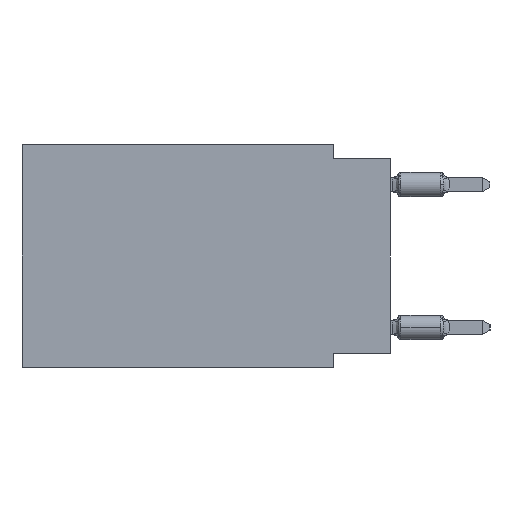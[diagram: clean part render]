
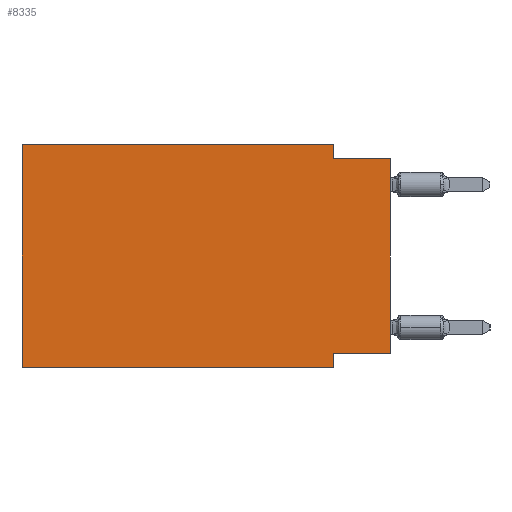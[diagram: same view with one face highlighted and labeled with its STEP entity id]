
A CAD part, left-side view. The second image highlights one B-rep face of the part: STEP entity #8335.
In plain terms, the highlighted planar face has unit normal (-1, 0, 0).
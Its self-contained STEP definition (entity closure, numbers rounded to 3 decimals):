
#845 = EDGE_CURVE ( 'NONE', #12443, #11943, #16083, .T. ) ;
#1323 = CARTESIAN_POINT ( 'NONE',  ( 0., 16.383, 0. ) ) ;
#2294 = EDGE_CURVE ( 'NONE', #23353, #10961, #6311, .T. ) ;
#3761 = VECTOR ( 'NONE', #19683, 1000. ) ;
#4020 = EDGE_CURVE ( 'NONE', #7304, #17691, #24039, .T. ) ;
#4338 = VECTOR ( 'NONE', #15937, 1000. ) ;
#4345 = EDGE_CURVE ( 'NONE', #23353, #12443, #23044, .T. ) ;
#4867 = CARTESIAN_POINT ( 'NONE',  ( 0., 2.54, -9.906 ) ) ;
#4906 = LINE ( 'NONE', #21512, #3761 ) ;
#5640 = EDGE_CURVE ( 'NONE', #17691, #22549, #6703, .T. ) ;
#6203 = ORIENTED_EDGE ( 'NONE', *, *, #845, .F. ) ;
#6311 = LINE ( 'NONE', #9970, #8726 ) ;
#6531 = EDGE_CURVE ( 'NONE', #10231, #10961, #4906, .T. ) ;
#6579 = ORIENTED_EDGE ( 'NONE', *, *, #4345, .F. ) ;
#6703 = LINE ( 'NONE', #17707, #21870 ) ;
#7304 = VERTEX_POINT ( 'NONE', #21574 ) ;
#8269 = ORIENTED_EDGE ( 'NONE', *, *, #5640, .F. ) ;
#8335 = ADVANCED_FACE ( 'NONE', ( #10735 ), #21973, .F. ) ;
#8495 = CARTESIAN_POINT ( 'NONE',  ( 0., 0., -9.271 ) ) ;
#8531 = AXIS2_PLACEMENT_3D ( 'NONE', #1323, #19904, #20152 ) ;
#8726 = VECTOR ( 'NONE', #17431, 1000. ) ;
#8880 = DIRECTION ( 'NONE',  ( 0., 0., 1. ) ) ;
#9063 = VECTOR ( 'NONE', #19872, 1000. ) ;
#9106 = EDGE_CURVE ( 'NONE', #7304, #11943, #16672, .T. ) ;
#9144 = EDGE_LOOP ( 'NONE', ( #17101, #19154, #11275, #8269, #10000, #17847, #6203, #6579 ) ) ;
#9970 = CARTESIAN_POINT ( 'NONE',  ( 0., 0., 0. ) ) ;
#10000 = ORIENTED_EDGE ( 'NONE', *, *, #4020, .F. ) ;
#10231 = VERTEX_POINT ( 'NONE', #10335 ) ;
#10335 = CARTESIAN_POINT ( 'NONE',  ( 0., 2.54, -0.635 ) ) ;
#10477 = DIRECTION ( 'NONE',  ( 0., -1., 0. ) ) ;
#10491 = CARTESIAN_POINT ( 'NONE',  ( 0., 16.383, 0. ) ) ;
#10735 = FACE_OUTER_BOUND ( 'NONE', #9144, .T. ) ;
#10957 = CARTESIAN_POINT ( 'NONE',  ( 0., 0., -9.271 ) ) ;
#10961 = VERTEX_POINT ( 'NONE', #11374 ) ;
#11225 = CARTESIAN_POINT ( 'NONE',  ( 0., 2.54, -9.271 ) ) ;
#11275 = ORIENTED_EDGE ( 'NONE', *, *, #22715, .F. ) ;
#11374 = CARTESIAN_POINT ( 'NONE',  ( 0., 0., -0.635 ) ) ;
#11943 = VERTEX_POINT ( 'NONE', #14064 ) ;
#12443 = VERTEX_POINT ( 'NONE', #11225 ) ;
#14064 = CARTESIAN_POINT ( 'NONE',  ( 0., 2.54, -9.906 ) ) ;
#14437 = VECTOR ( 'NONE', #8880, 1000. ) ;
#14711 = CARTESIAN_POINT ( 'NONE',  ( 0., 16.383, 0. ) ) ;
#15826 = VECTOR ( 'NONE', #23129, 1000. ) ;
#15937 = DIRECTION ( 'NONE',  ( 0., 1., 0. ) ) ;
#16083 = LINE ( 'NONE', #4867, #9063 ) ;
#16294 = DIRECTION ( 'NONE',  ( 0., -1., 0. ) ) ;
#16672 = LINE ( 'NONE', #24128, #24131 ) ;
#17101 = ORIENTED_EDGE ( 'NONE', *, *, #2294, .T. ) ;
#17431 = DIRECTION ( 'NONE',  ( 0., 0., 1. ) ) ;
#17691 = VERTEX_POINT ( 'NONE', #10491 ) ;
#17707 = CARTESIAN_POINT ( 'NONE',  ( 0., 16.383, 0. ) ) ;
#17847 = ORIENTED_EDGE ( 'NONE', *, *, #9106, .T. ) ;
#18853 = CARTESIAN_POINT ( 'NONE',  ( 0., 2.54, 0. ) ) ;
#19154 = ORIENTED_EDGE ( 'NONE', *, *, #6531, .F. ) ;
#19683 = DIRECTION ( 'NONE',  ( 0., -1., 0. ) ) ;
#19872 = DIRECTION ( 'NONE',  ( 0., 0., -1. ) ) ;
#19904 = DIRECTION ( 'NONE',  ( 1., 0., 0. ) ) ;
#20152 = DIRECTION ( 'NONE',  ( 0., 0., -1. ) ) ;
#21178 = LINE ( 'NONE', #21296, #15826 ) ;
#21296 = CARTESIAN_POINT ( 'NONE',  ( 0., 2.54, 0. ) ) ;
#21512 = CARTESIAN_POINT ( 'NONE',  ( 0., 0., -0.635 ) ) ;
#21574 = CARTESIAN_POINT ( 'NONE',  ( 0., 16.383, -9.906 ) ) ;
#21870 = VECTOR ( 'NONE', #10477, 1000. ) ;
#21973 = PLANE ( 'NONE',  #8531 ) ;
#22549 = VERTEX_POINT ( 'NONE', #18853 ) ;
#22715 = EDGE_CURVE ( 'NONE', #22549, #10231, #21178, .T. ) ;
#23044 = LINE ( 'NONE', #8495, #4338 ) ;
#23129 = DIRECTION ( 'NONE',  ( 0., 0., -1. ) ) ;
#23353 = VERTEX_POINT ( 'NONE', #10957 ) ;
#24039 = LINE ( 'NONE', #14711, #14437 ) ;
#24128 = CARTESIAN_POINT ( 'NONE',  ( 0., 16.383, -9.906 ) ) ;
#24131 = VECTOR ( 'NONE', #16294, 1000. ) ;
